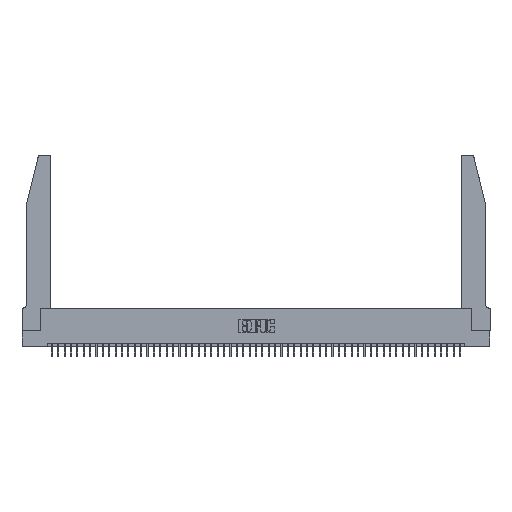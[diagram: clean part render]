
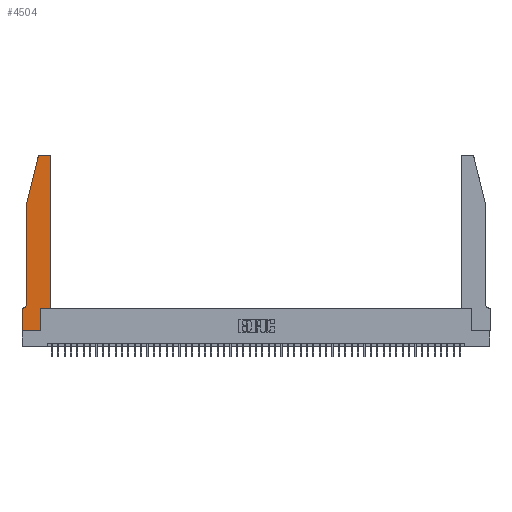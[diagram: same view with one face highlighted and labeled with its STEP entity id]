
A CAD part, top view. The second image highlights one B-rep face of the part: STEP entity #4504.
In plain terms, the highlighted planar face has unit normal (0, 0, 1).
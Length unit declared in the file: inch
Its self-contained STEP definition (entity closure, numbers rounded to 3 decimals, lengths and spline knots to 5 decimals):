
#634 = CARTESIAN_POINT ( 'NONE',  ( 0.2605, 2.75, 0.37 ) ) ;
#2829 = VECTOR ( 'NONE', #51843, 39.37008 ) ;
#2903 = FACE_OUTER_BOUND ( 'NONE', #20492, .T. ) ;
#3608 = VERTEX_POINT ( 'NONE', #49635 ) ;
#4487 = VERTEX_POINT ( 'NONE', #10094 ) ;
#4504 = ADVANCED_FACE ( 'NONE', ( #2903 ), #34646, .T. ) ;
#5772 = VERTEX_POINT ( 'NONE', #31681 ) ;
#6188 = AXIS2_PLACEMENT_3D ( 'NONE', #17653, #46093, #21807 ) ;
#6588 = VERTEX_POINT ( 'NONE', #34742 ) ;
#7496 = EDGE_CURVE ( 'NONE', #5772, #23043, #51571, .T. ) ;
#8361 = VECTOR ( 'NONE', #13937, 39.37008 ) ;
#8592 = EDGE_CURVE ( 'NONE', #52489, #44742, #21780, .T. ) ;
#8632 = VECTOR ( 'NONE', #29099, 39.37008 ) ;
#9481 = ORIENTED_EDGE ( 'NONE', *, *, #11642, .T. ) ;
#10094 = CARTESIAN_POINT ( 'NONE',  ( 0.4205, 2.75, 0.37 ) ) ;
#10280 = CARTESIAN_POINT ( 'NONE',  ( 0., 0.35, 0.37 ) ) ;
#10689 = LINE ( 'NONE', #41110, #50104 ) ;
#11642 = EDGE_CURVE ( 'NONE', #3608, #46988, #19466, .T. ) ;
#11843 = ORIENTED_EDGE ( 'NONE', *, *, #18496, .T. ) ;
#13937 = DIRECTION ( 'NONE',  ( 1., 0., 0. ) ) ;
#14388 = DIRECTION ( 'NONE',  ( 1., 0., 0. ) ) ;
#14498 = CARTESIAN_POINT ( 'NONE',  ( 0.284, 2.72, 0.37 ) ) ;
#14751 = ORIENTED_EDGE ( 'NONE', *, *, #7496, .T. ) ;
#14890 = ORIENTED_EDGE ( 'NONE', *, *, #34675, .T. ) ;
#15124 = DIRECTION ( 'NONE',  ( 0., -1., 0. ) ) ;
#17653 = CARTESIAN_POINT ( 'NONE',  ( 0.4205, 2.72, 0.37 ) ) ;
#18054 = VECTOR ( 'NONE', #15124, 39.37008 ) ;
#18265 = CARTESIAN_POINT ( 'NONE',  ( 0.0755, 0.42, 0.37 ) ) ;
#18496 = EDGE_CURVE ( 'NONE', #6588, #5772, #35361, .T. ) ;
#18577 = DIRECTION ( 'NONE',  ( 1., 0., 0. ) ) ;
#19069 = CARTESIAN_POINT ( 'NONE',  ( 0.4505, 2.72, 0.37 ) ) ;
#19466 = LINE ( 'NONE', #37062, #8632 ) ;
#20492 = EDGE_LOOP ( 'NONE', ( #49928, #32282, #9481, #48229, #39666, #37338, #39576, #11843, #14751, #23543, #14890, #24964 ) ) ;
#21780 = CIRCLE ( 'NONE', #29177, 0.07 ) ;
#21807 = DIRECTION ( 'NONE',  ( 1., 0., 0. ) ) ;
#22004 = DIRECTION ( 'NONE',  ( 0., 1., 0. ) ) ;
#22164 = VECTOR ( 'NONE', #22004, 39.37008 ) ;
#22856 = CARTESIAN_POINT ( 'NONE',  ( 0.0055, 0.42, 0.37 ) ) ;
#22930 = AXIS2_PLACEMENT_3D ( 'NONE', #14498, #42935, #18577 ) ;
#23043 = VERTEX_POINT ( 'NONE', #38050 ) ;
#23543 = ORIENTED_EDGE ( 'NONE', *, *, #37865, .T. ) ;
#23640 = CARTESIAN_POINT ( 'NONE',  ( 0.0055, 0.35, 0.37 ) ) ;
#24223 = CIRCLE ( 'NONE', #22930, 0.03 ) ;
#24964 = ORIENTED_EDGE ( 'NONE', *, *, #30219, .T. ) ;
#25342 = VERTEX_POINT ( 'NONE', #19069 ) ;
#25487 = EDGE_CURVE ( 'NONE', #47250, #6588, #10689, .T. ) ;
#25810 = AXIS2_PLACEMENT_3D ( 'NONE', #10280, #38724, #14388 ) ;
#26946 = DIRECTION ( 'NONE',  ( -1., 0., 0. ) ) ;
#28181 = VERTEX_POINT ( 'NONE', #37202 ) ;
#28517 = LINE ( 'NONE', #634, #29799 ) ;
#28908 = LINE ( 'NONE', #39498, #18054 ) ;
#29099 = DIRECTION ( 'NONE',  ( -0.239, -0.971, 0. ) ) ;
#29177 = AXIS2_PLACEMENT_3D ( 'NONE', #22856, #51193, #26946 ) ;
#29278 = DIRECTION ( 'NONE',  ( -1., 0., 0. ) ) ;
#29799 = VECTOR ( 'NONE', #29278, 39.37008 ) ;
#30219 = EDGE_CURVE ( 'NONE', #25342, #4487, #36880, .T. ) ;
#31667 = LINE ( 'NONE', #46302, #22164 ) ;
#31681 = CARTESIAN_POINT ( 'NONE',  ( 0.2865, 0., 0.37 ) ) ;
#32249 = CARTESIAN_POINT ( 'NONE',  ( 0.284, 2.75, 0.37 ) ) ;
#32282 = ORIENTED_EDGE ( 'NONE', *, *, #47996, .T. ) ;
#32585 = LINE ( 'NONE', #42393, #8361 ) ;
#33812 = DIRECTION ( 'NONE',  ( 0., 1., 0. ) ) ;
#34526 = EDGE_CURVE ( 'NONE', #4487, #44059, #28517, .T. ) ;
#34646 = PLANE ( 'NONE',  #25810 ) ;
#34675 = EDGE_CURVE ( 'NONE', #28181, #25342, #31667, .T. ) ;
#34742 = CARTESIAN_POINT ( 'NONE',  ( 0., 0., 0.37 ) ) ;
#35361 = LINE ( 'NONE', #35555, #2829 ) ;
#35555 = CARTESIAN_POINT ( 'NONE',  ( 0., 0., 0.37 ) ) ;
#36880 = CIRCLE ( 'NONE', #6188, 0.03 ) ;
#37062 = CARTESIAN_POINT ( 'NONE',  ( 0.0755, 2., 0.37 ) ) ;
#37202 = CARTESIAN_POINT ( 'NONE',  ( 0.4505, 0.35, 0.37 ) ) ;
#37338 = ORIENTED_EDGE ( 'NONE', *, *, #40150, .T. ) ;
#37865 = EDGE_CURVE ( 'NONE', #23043, #28181, #32585, .T. ) ;
#38050 = CARTESIAN_POINT ( 'NONE',  ( 0.2865, 0.35, 0.37 ) ) ;
#38699 = LINE ( 'NONE', #39885, #46963 ) ;
#38724 = DIRECTION ( 'NONE',  ( 0., 0., 1. ) ) ;
#39498 = CARTESIAN_POINT ( 'NONE',  ( 0.0755, 2., 0.37 ) ) ;
#39576 = ORIENTED_EDGE ( 'NONE', *, *, #25487, .T. ) ;
#39666 = ORIENTED_EDGE ( 'NONE', *, *, #8592, .T. ) ;
#39885 = CARTESIAN_POINT ( 'NONE',  ( 0.0755, 0.35, 0.37 ) ) ;
#40150 = EDGE_CURVE ( 'NONE', #44742, #47250, #38699, .T. ) ;
#41110 = CARTESIAN_POINT ( 'NONE',  ( 0., 0., 0.37 ) ) ;
#42393 = CARTESIAN_POINT ( 'NONE',  ( 0.4505, 0.35, 0.37 ) ) ;
#42935 = DIRECTION ( 'NONE',  ( 0., 0., 1. ) ) ;
#43977 = DIRECTION ( 'NONE',  ( -1., 0., 0. ) ) ;
#44059 = VERTEX_POINT ( 'NONE', #32249 ) ;
#44742 = VERTEX_POINT ( 'NONE', #23640 ) ;
#45029 = DIRECTION ( 'NONE',  ( 0., -1., 0. ) ) ;
#45891 = CARTESIAN_POINT ( 'NONE',  ( 0.2865, 0.35, 0.37 ) ) ;
#45895 = EDGE_CURVE ( 'NONE', #46988, #52489, #28908, .T. ) ;
#46093 = DIRECTION ( 'NONE',  ( 0., 0., 1. ) ) ;
#46302 = CARTESIAN_POINT ( 'NONE',  ( 0.4505, 0.35, 0.37 ) ) ;
#46963 = VECTOR ( 'NONE', #43977, 39.37008 ) ;
#46988 = VERTEX_POINT ( 'NONE', #50376 ) ;
#47250 = VERTEX_POINT ( 'NONE', #52072 ) ;
#47996 = EDGE_CURVE ( 'NONE', #44059, #3608, #24223, .T. ) ;
#48229 = ORIENTED_EDGE ( 'NONE', *, *, #45895, .T. ) ;
#49635 = CARTESIAN_POINT ( 'NONE',  ( 0.25487, 2.72718, 0.37 ) ) ;
#49928 = ORIENTED_EDGE ( 'NONE', *, *, #34526, .T. ) ;
#50104 = VECTOR ( 'NONE', #45029, 39.37008 ) ;
#50335 = VECTOR ( 'NONE', #33812, 39.37008 ) ;
#50376 = CARTESIAN_POINT ( 'NONE',  ( 0.0755, 2., 0.37 ) ) ;
#51193 = DIRECTION ( 'NONE',  ( 0., 0., -1. ) ) ;
#51571 = LINE ( 'NONE', #45891, #50335 ) ;
#51843 = DIRECTION ( 'NONE',  ( 1., 0., 0. ) ) ;
#52072 = CARTESIAN_POINT ( 'NONE',  ( 0., 0.35, 0.37 ) ) ;
#52489 = VERTEX_POINT ( 'NONE', #18265 ) ;
